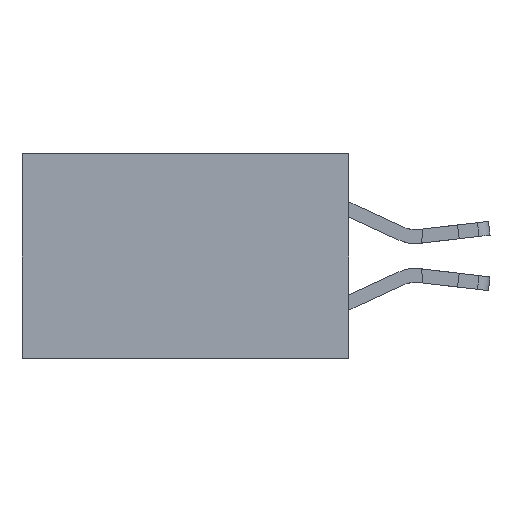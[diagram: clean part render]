
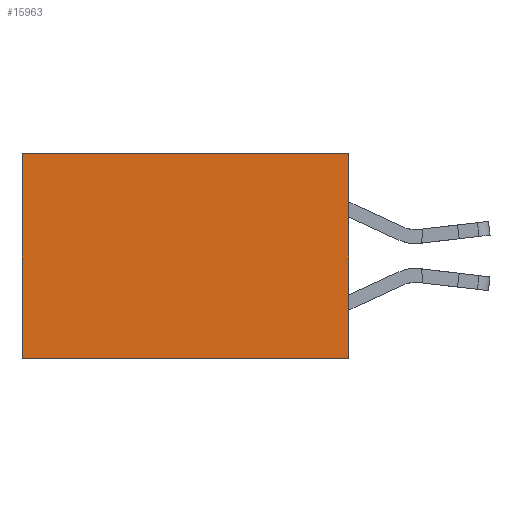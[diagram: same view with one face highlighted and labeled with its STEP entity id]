
A CAD part, left-side view. The second image highlights one B-rep face of the part: STEP entity #15963.
In plain terms, the highlighted planar face has unit normal (-1, 0, 0).
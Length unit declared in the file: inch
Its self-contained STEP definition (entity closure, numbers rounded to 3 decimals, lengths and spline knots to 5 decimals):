
#1334 = LINE ( 'NONE', #11195, #9780 ) ;
#1357 = CARTESIAN_POINT ( 'NONE',  ( 0.277, 0.59, 0. ) ) ;
#2408 = VECTOR ( 'NONE', #10304, 39.37008 ) ;
#2592 = VECTOR ( 'NONE', #12935, 39.37008 ) ;
#2755 = EDGE_LOOP ( 'NONE', ( #8606, #13386, #17708, #9612 ) ) ;
#2866 = AXIS2_PLACEMENT_3D ( 'NONE', #14090, #17351, #7654 ) ;
#2912 = DIRECTION ( 'NONE',  ( 0., 0., -1. ) ) ;
#5715 = VECTOR ( 'NONE', #19597, 39.37008 ) ;
#5881 = EDGE_CURVE ( 'NONE', #7177, #17106, #15215, .T. ) ;
#7177 = VERTEX_POINT ( 'NONE', #18806 ) ;
#7467 = LINE ( 'NONE', #13590, #2408 ) ;
#7654 = DIRECTION ( 'NONE',  ( 0., 0., -1. ) ) ;
#8218 = CARTESIAN_POINT ( 'NONE',  ( 0.277, 0., -0.37 ) ) ;
#8606 = ORIENTED_EDGE ( 'NONE', *, *, #19949, .T. ) ;
#9025 = VERTEX_POINT ( 'NONE', #18255 ) ;
#9612 = ORIENTED_EDGE ( 'NONE', *, *, #5881, .T. ) ;
#9780 = VECTOR ( 'NONE', #2912, 39.37008 ) ;
#10304 = DIRECTION ( 'NONE',  ( 0., 1., 0. ) ) ;
#11195 = CARTESIAN_POINT ( 'NONE',  ( 0.277, 0.59, -0.37 ) ) ;
#12935 = DIRECTION ( 'NONE',  ( 0., 1., 0. ) ) ;
#13386 = ORIENTED_EDGE ( 'NONE', *, *, #19619, .F. ) ;
#13411 = CARTESIAN_POINT ( 'NONE',  ( 0.277, 0., 0. ) ) ;
#13590 = CARTESIAN_POINT ( 'NONE',  ( 0.277, 0., -0.37 ) ) ;
#14090 = CARTESIAN_POINT ( 'NONE',  ( 0.277, 0., -0.37 ) ) ;
#14323 = EDGE_CURVE ( 'NONE', #7177, #15973, #18695, .T. ) ;
#15215 = LINE ( 'NONE', #13411, #2592 ) ;
#15963 = ADVANCED_FACE ( 'NONE', ( #17358 ), #20531, .F. ) ;
#15973 = VERTEX_POINT ( 'NONE', #20599 ) ;
#17106 = VERTEX_POINT ( 'NONE', #1357 ) ;
#17351 = DIRECTION ( 'NONE',  ( 1., 0., 0. ) ) ;
#17358 = FACE_OUTER_BOUND ( 'NONE', #2755, .T. ) ;
#17708 = ORIENTED_EDGE ( 'NONE', *, *, #14323, .F. ) ;
#18255 = CARTESIAN_POINT ( 'NONE',  ( 0.277, 0.59, -0.37 ) ) ;
#18695 = LINE ( 'NONE', #8218, #5715 ) ;
#18806 = CARTESIAN_POINT ( 'NONE',  ( 0.277, 0., 0. ) ) ;
#19597 = DIRECTION ( 'NONE',  ( 0., 0., -1. ) ) ;
#19619 = EDGE_CURVE ( 'NONE', #15973, #9025, #7467, .T. ) ;
#19949 = EDGE_CURVE ( 'NONE', #17106, #9025, #1334, .T. ) ;
#20531 = PLANE ( 'NONE',  #2866 ) ;
#20599 = CARTESIAN_POINT ( 'NONE',  ( 0.277, 0., -0.37 ) ) ;
